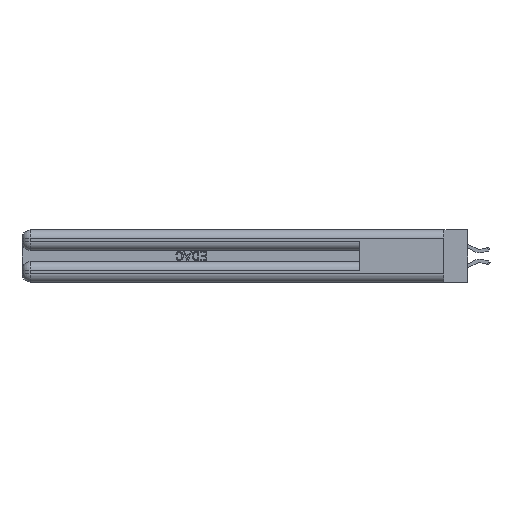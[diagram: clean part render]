
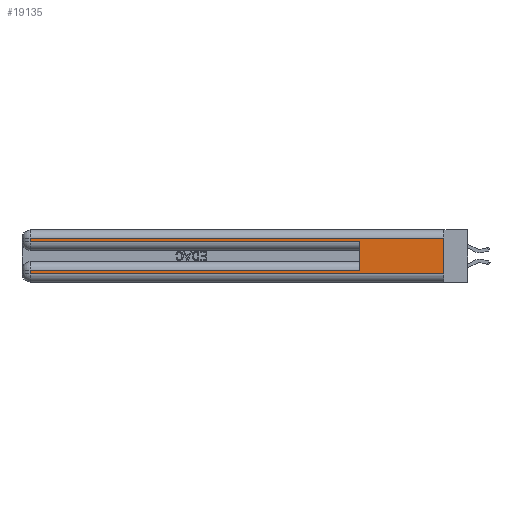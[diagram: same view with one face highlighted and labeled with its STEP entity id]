
A CAD part, left-side view. The second image highlights one B-rep face of the part: STEP entity #19135.
In plain terms, the highlighted planar face has unit normal (-1, 0, 0).
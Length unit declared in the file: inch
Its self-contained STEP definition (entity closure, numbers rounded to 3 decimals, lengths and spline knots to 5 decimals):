
#177 = VERTEX_POINT ( 'NONE', #19091 ) ;
#2533 = CARTESIAN_POINT ( 'NONE',  ( 0., 2.94, 0.31 ) ) ;
#2749 = CARTESIAN_POINT ( 'NONE',  ( 0., 2.94, 0.37 ) ) ;
#3897 = CARTESIAN_POINT ( 'NONE',  ( 0., 2.94, 0.085 ) ) ;
#6084 = CARTESIAN_POINT ( 'NONE',  ( 0., 0., 0.06 ) ) ;
#6322 = ORIENTED_EDGE ( 'NONE', *, *, #22601, .T. ) ;
#6580 = DIRECTION ( 'NONE',  ( 0., 0., -1. ) ) ;
#6830 = VECTOR ( 'NONE', #40394, 39.37008 ) ;
#7180 = VERTEX_POINT ( 'NONE', #2533 ) ;
#7410 = VECTOR ( 'NONE', #6580, 39.37008 ) ;
#8142 = VERTEX_POINT ( 'NONE', #9097 ) ;
#8611 = LINE ( 'NONE', #2749, #7410 ) ;
#9097 = CARTESIAN_POINT ( 'NONE',  ( 0., 0., 0.31 ) ) ;
#10133 = VECTOR ( 'NONE', #16179, 39.37008 ) ;
#10244 = CARTESIAN_POINT ( 'NONE',  ( 0., 0.6, 0.145 ) ) ;
#10825 = ORIENTED_EDGE ( 'NONE', *, *, #17985, .T. ) ;
#10883 = VECTOR ( 'NONE', #13225, 39.37008 ) ;
#11911 = CARTESIAN_POINT ( 'NONE',  ( 0., 0., 0.31 ) ) ;
#12365 = CARTESIAN_POINT ( 'NONE',  ( 0., 2.94, 0.37 ) ) ;
#13225 = DIRECTION ( 'NONE',  ( 0., -1., 0. ) ) ;
#14358 = LINE ( 'NONE', #12365, #10133 ) ;
#14451 = EDGE_CURVE ( 'NONE', #8142, #25489, #45435, .T. ) ;
#16179 = DIRECTION ( 'NONE',  ( 0., 0., -1. ) ) ;
#17985 = EDGE_CURVE ( 'NONE', #177, #38598, #22109, .T. ) ;
#18261 = CARTESIAN_POINT ( 'NONE',  ( 0., 0.6, 0.085 ) ) ;
#19091 = CARTESIAN_POINT ( 'NONE',  ( 0., 2.94, 0.285 ) ) ;
#19135 = ADVANCED_FACE ( 'NONE', ( #31468 ), #20911, .F. ) ;
#19150 = CARTESIAN_POINT ( 'NONE',  ( 0., 0., 0.37 ) ) ;
#20911 = PLANE ( 'NONE',  #42497 ) ;
#22109 = LINE ( 'NONE', #43376, #10883 ) ;
#22321 = CARTESIAN_POINT ( 'NONE',  ( 0., 2.94, 0.06 ) ) ;
#22601 = EDGE_CURVE ( 'NONE', #7180, #177, #8611, .T. ) ;
#22963 = DIRECTION ( 'NONE',  ( 0., 0., -1. ) ) ;
#24896 = DIRECTION ( 'NONE',  ( 0., 0., -1. ) ) ;
#24932 = ORIENTED_EDGE ( 'NONE', *, *, #45507, .T. ) ;
#25290 = DIRECTION ( 'NONE',  ( 0., 1., 0. ) ) ;
#25462 = VECTOR ( 'NONE', #22963, 39.37008 ) ;
#25489 = VERTEX_POINT ( 'NONE', #40748 ) ;
#26412 = ORIENTED_EDGE ( 'NONE', *, *, #14451, .F. ) ;
#29276 = EDGE_CURVE ( 'NONE', #35363, #34703, #14358, .T. ) ;
#31314 = ORIENTED_EDGE ( 'NONE', *, *, #41413, .F. ) ;
#31468 = FACE_OUTER_BOUND ( 'NONE', #40704, .T. ) ;
#34456 = VECTOR ( 'NONE', #25290, 39.37008 ) ;
#34703 = VERTEX_POINT ( 'NONE', #22321 ) ;
#34876 = VECTOR ( 'NONE', #42056, 39.37008 ) ;
#35041 = EDGE_CURVE ( 'NONE', #34703, #25489, #46698, .T. ) ;
#35363 = VERTEX_POINT ( 'NONE', #3897 ) ;
#36057 = LINE ( 'NONE', #11911, #34876 ) ;
#36739 = VECTOR ( 'NONE', #40056, 39.37008 ) ;
#38151 = LINE ( 'NONE', #10244, #6830 ) ;
#38598 = VERTEX_POINT ( 'NONE', #44255 ) ;
#38664 = VERTEX_POINT ( 'NONE', #18261 ) ;
#39815 = CARTESIAN_POINT ( 'NONE',  ( 0., 0., 0.37 ) ) ;
#40056 = DIRECTION ( 'NONE',  ( 0., -1., 0. ) ) ;
#40394 = DIRECTION ( 'NONE',  ( 0., 0., 1. ) ) ;
#40704 = EDGE_LOOP ( 'NONE', ( #26412, #24932, #6322, #10825, #31314, #42902, #42025, #44343 ) ) ;
#40748 = CARTESIAN_POINT ( 'NONE',  ( 0., 0., 0.06 ) ) ;
#41413 = EDGE_CURVE ( 'NONE', #38664, #38598, #38151, .T. ) ;
#42025 = ORIENTED_EDGE ( 'NONE', *, *, #29276, .T. ) ;
#42056 = DIRECTION ( 'NONE',  ( 0., 1., 0. ) ) ;
#42497 = AXIS2_PLACEMENT_3D ( 'NONE', #39815, #47355, #24896 ) ;
#42902 = ORIENTED_EDGE ( 'NONE', *, *, #43929, .T. ) ;
#43376 = CARTESIAN_POINT ( 'NONE',  ( 0., 0., 0.285 ) ) ;
#43929 = EDGE_CURVE ( 'NONE', #38664, #35363, #44416, .T. ) ;
#43974 = CARTESIAN_POINT ( 'NONE',  ( 0., 0., 0.085 ) ) ;
#44255 = CARTESIAN_POINT ( 'NONE',  ( 0., 0.6, 0.285 ) ) ;
#44343 = ORIENTED_EDGE ( 'NONE', *, *, #35041, .T. ) ;
#44416 = LINE ( 'NONE', #43974, #34456 ) ;
#45435 = LINE ( 'NONE', #19150, #25462 ) ;
#45507 = EDGE_CURVE ( 'NONE', #8142, #7180, #36057, .T. ) ;
#46698 = LINE ( 'NONE', #6084, #36739 ) ;
#47355 = DIRECTION ( 'NONE',  ( 1., 0., 0. ) ) ;
